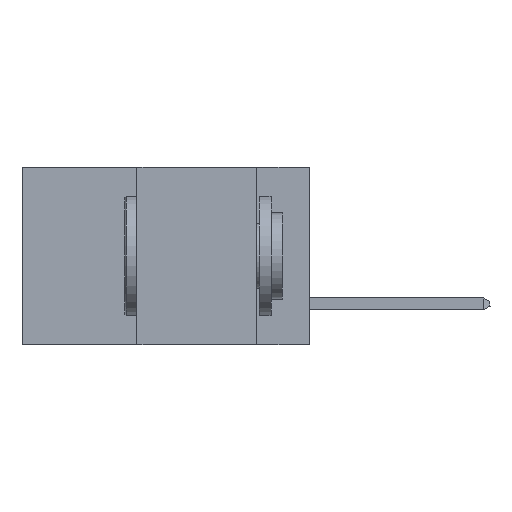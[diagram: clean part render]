
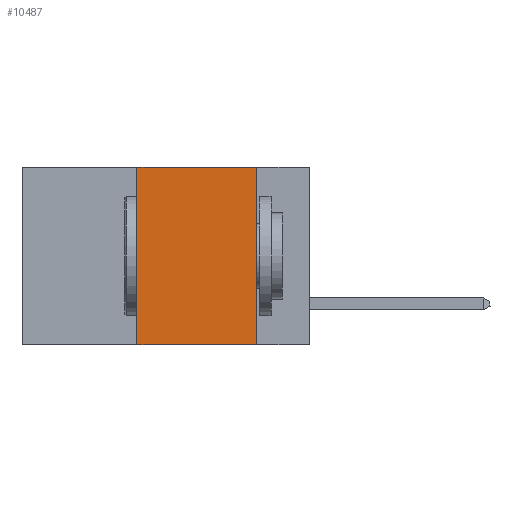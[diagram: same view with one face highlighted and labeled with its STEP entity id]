
A CAD part, left-side view. The second image highlights one B-rep face of the part: STEP entity #10487.
In plain terms, the highlighted planar face has unit normal (-1, 0, 0).
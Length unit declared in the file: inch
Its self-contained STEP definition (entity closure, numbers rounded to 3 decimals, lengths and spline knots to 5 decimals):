
#1204 = LINE ( 'NONE', #13733, #8576 ) ;
#1586 = CARTESIAN_POINT ( 'NONE',  ( 0., 0.11, 0. ) ) ;
#1939 = LINE ( 'NONE', #12560, #18022 ) ;
#3261 = VERTEX_POINT ( 'NONE', #7017 ) ;
#3593 = CARTESIAN_POINT ( 'NONE',  ( 0., 0.36, -0.37 ) ) ;
#3861 = CARTESIAN_POINT ( 'NONE',  ( 0., 0.36, 0. ) ) ;
#4069 = DIRECTION ( 'NONE',  ( 1., 0., 0. ) ) ;
#4260 = CARTESIAN_POINT ( 'NONE',  ( 0., 0.11, -0.37 ) ) ;
#4485 = DIRECTION ( 'NONE',  ( 0., -1., 0. ) ) ;
#4553 = ORIENTED_EDGE ( 'NONE', *, *, #20000, .F. ) ;
#4940 = ORIENTED_EDGE ( 'NONE', *, *, #18980, .F. ) ;
#5071 = ORIENTED_EDGE ( 'NONE', *, *, #17952, .T. ) ;
#5210 = LINE ( 'NONE', #3861, #17848 ) ;
#5619 = VECTOR ( 'NONE', #4485, 39.37008 ) ;
#5638 = DIRECTION ( 'NONE',  ( 0., 0., 1. ) ) ;
#5703 = EDGE_CURVE ( 'NONE', #3261, #17010, #1939, .T. ) ;
#6404 = ORIENTED_EDGE ( 'NONE', *, *, #5703, .F. ) ;
#7017 = CARTESIAN_POINT ( 'NONE',  ( 0., 0.36, 0. ) ) ;
#7418 = PLANE ( 'NONE',  #16752 ) ;
#8576 = VECTOR ( 'NONE', #15381, 39.37008 ) ;
#8698 = VERTEX_POINT ( 'NONE', #4260 ) ;
#9475 = CARTESIAN_POINT ( 'NONE',  ( 0., 0.6, -0.37 ) ) ;
#10487 = ADVANCED_FACE ( 'NONE', ( #14018 ), #7418, .F. ) ;
#10910 = DIRECTION ( 'NONE',  ( 0., -1., 0. ) ) ;
#12560 = CARTESIAN_POINT ( 'NONE',  ( 0., 0.6, 0. ) ) ;
#13733 = CARTESIAN_POINT ( 'NONE',  ( 0., 0.11, 0. ) ) ;
#14018 = FACE_OUTER_BOUND ( 'NONE', #19592, .T. ) ;
#14073 = CARTESIAN_POINT ( 'NONE',  ( 0., 0.6, 0. ) ) ;
#14862 = VERTEX_POINT ( 'NONE', #3593 ) ;
#15381 = DIRECTION ( 'NONE',  ( 0., 0., -1. ) ) ;
#15716 = DIRECTION ( 'NONE',  ( 0., 0., -1. ) ) ;
#16752 = AXIS2_PLACEMENT_3D ( 'NONE', #14073, #4069, #15716 ) ;
#17010 = VERTEX_POINT ( 'NONE', #1586 ) ;
#17848 = VECTOR ( 'NONE', #5638, 39.37008 ) ;
#17952 = EDGE_CURVE ( 'NONE', #14862, #8698, #19170, .T. ) ;
#18022 = VECTOR ( 'NONE', #10910, 39.37008 ) ;
#18980 = EDGE_CURVE ( 'NONE', #14862, #3261, #5210, .T. ) ;
#19170 = LINE ( 'NONE', #9475, #5619 ) ;
#19592 = EDGE_LOOP ( 'NONE', ( #4553, #6404, #4940, #5071 ) ) ;
#20000 = EDGE_CURVE ( 'NONE', #17010, #8698, #1204, .T. ) ;
